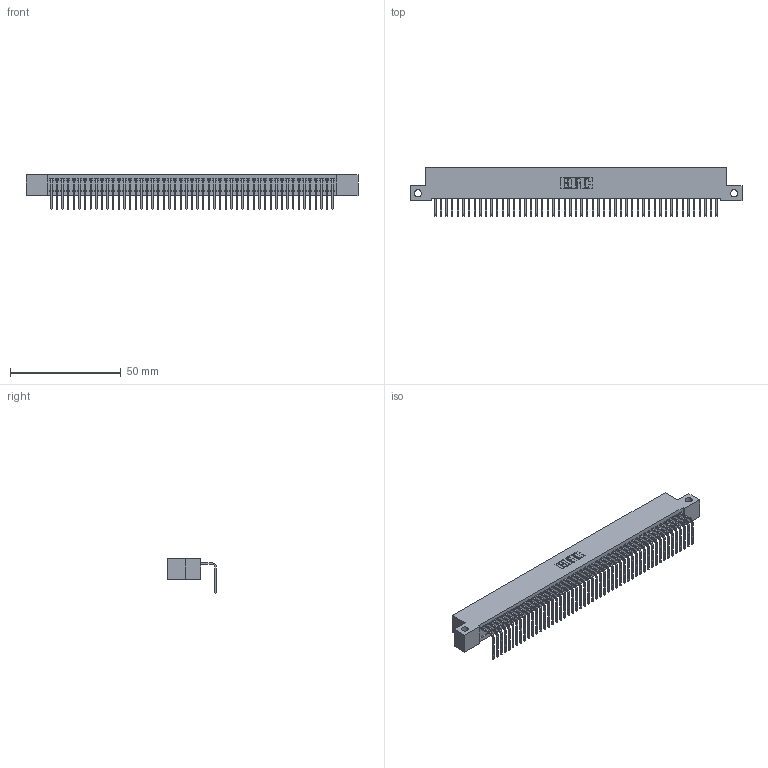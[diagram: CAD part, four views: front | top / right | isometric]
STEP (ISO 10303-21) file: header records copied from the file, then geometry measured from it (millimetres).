
FILE_DESCRIPTION (( 'STEP AP203' ), '1' );
FILE_NAME ('342-051-558-112.STEP', '2018-08-12T21:12:10', ( '' ), ( '' ), 'SwSTEP 2.0', 'SolidWorks 2016', '' );
FILE_SCHEMA (( 'CONFIG_CONTROL_DESIGN' ));
Length unit declared in the file: inch
Products named in the file (3): 342 Part_Side Mount; 345-292-001_558 Tail - 2; 342-051-558-112
Assembly tree (52 placements, depth 2):
  342-051-558-112
    342 Part_Side Mount
    345-292-001_558 Tail - 2  x51
Bounding box: 149.86 x 21.91 x 15.62 mm (x, y, z)
Volume: 13268.9 mm3; surface area: 20454.7 mm2
Topology: 52 solids, 52 shells, 3170 faces, 9581 edges, 6318 vertices
Faces by surface type: plane 2310, cylinder 860
Entity records: 29969 total; most frequent: CARTESIAN_POINT 5175, ORIENTED_EDGE 5162, DIRECTION 4347, EDGE_CURVE 2581, VECTOR 2453, LINE 2453, VERTEX_POINT 1718, AXIS2_PLACEMENT_3D 947
